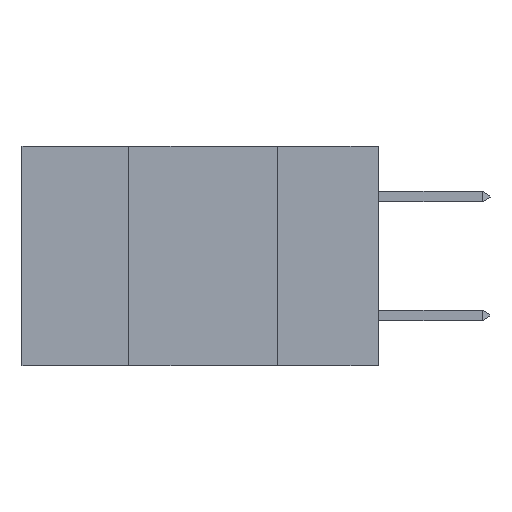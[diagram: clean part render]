
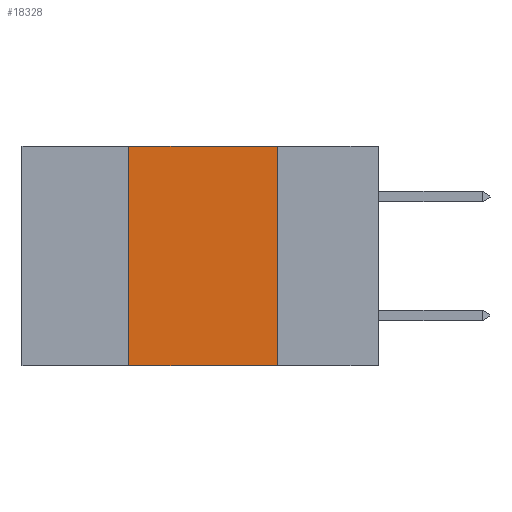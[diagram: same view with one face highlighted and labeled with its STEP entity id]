
A CAD part, left-side view. The second image highlights one B-rep face of the part: STEP entity #18328.
In plain terms, the highlighted planar face has unit normal (-1, 0, 0).
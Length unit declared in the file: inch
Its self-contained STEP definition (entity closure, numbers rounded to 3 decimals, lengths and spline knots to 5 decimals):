
#349 = LINE ( 'NONE', #16139, #8867 ) ;
#1029 = CARTESIAN_POINT ( 'NONE',  ( 0., 0.42, 0. ) ) ;
#1125 = AXIS2_PLACEMENT_3D ( 'NONE', #12153, #16724, #7629 ) ;
#2947 = EDGE_CURVE ( 'NONE', #4240, #19708, #18165, .T. ) ;
#3230 = VERTEX_POINT ( 'NONE', #1029 ) ;
#3625 = CARTESIAN_POINT ( 'NONE',  ( 0., 0.17, -0.37 ) ) ;
#4240 = VERTEX_POINT ( 'NONE', #11007 ) ;
#5170 = EDGE_CURVE ( 'NONE', #18946, #3230, #349, .T. ) ;
#7629 = DIRECTION ( 'NONE',  ( 0., 0., -1. ) ) ;
#8013 = VECTOR ( 'NONE', #11892, 39.37008 ) ;
#8538 = EDGE_CURVE ( 'NONE', #18946, #19708, #20513, .T. ) ;
#8867 = VECTOR ( 'NONE', #19160, 39.37008 ) ;
#9620 = VECTOR ( 'NONE', #17182, 39.37008 ) ;
#11007 = CARTESIAN_POINT ( 'NONE',  ( 0., 0.17, 0. ) ) ;
#11129 = ORIENTED_EDGE ( 'NONE', *, *, #8538, .T. ) ;
#11775 = EDGE_CURVE ( 'NONE', #3230, #4240, #16071, .T. ) ;
#11892 = DIRECTION ( 'NONE',  ( 0., -1., 0. ) ) ;
#12153 = CARTESIAN_POINT ( 'NONE',  ( 0., 0.6, 0. ) ) ;
#12509 = VECTOR ( 'NONE', #17464, 39.37008 ) ;
#13045 = ORIENTED_EDGE ( 'NONE', *, *, #2947, .F. ) ;
#13361 = CARTESIAN_POINT ( 'NONE',  ( 0., 0.6, 0. ) ) ;
#14089 = EDGE_LOOP ( 'NONE', ( #13045, #15999, #15626, #11129 ) ) ;
#15161 = PLANE ( 'NONE',  #1125 ) ;
#15262 = CARTESIAN_POINT ( 'NONE',  ( 0., 0.17, 0. ) ) ;
#15626 = ORIENTED_EDGE ( 'NONE', *, *, #5170, .F. ) ;
#15909 = CARTESIAN_POINT ( 'NONE',  ( 0., 0.6, -0.37 ) ) ;
#15999 = ORIENTED_EDGE ( 'NONE', *, *, #11775, .F. ) ;
#16071 = LINE ( 'NONE', #13361, #8013 ) ;
#16139 = CARTESIAN_POINT ( 'NONE',  ( 0., 0.42, 0. ) ) ;
#16198 = CARTESIAN_POINT ( 'NONE',  ( 0., 0.42, -0.37 ) ) ;
#16724 = DIRECTION ( 'NONE',  ( 1., 0., 0. ) ) ;
#17182 = DIRECTION ( 'NONE',  ( 0., 0., -1. ) ) ;
#17464 = DIRECTION ( 'NONE',  ( 0., -1., 0. ) ) ;
#18165 = LINE ( 'NONE', #15262, #9620 ) ;
#18328 = ADVANCED_FACE ( 'NONE', ( #19063 ), #15161, .F. ) ;
#18946 = VERTEX_POINT ( 'NONE', #16198 ) ;
#19063 = FACE_OUTER_BOUND ( 'NONE', #14089, .T. ) ;
#19160 = DIRECTION ( 'NONE',  ( 0., 0., 1. ) ) ;
#19708 = VERTEX_POINT ( 'NONE', #3625 ) ;
#20513 = LINE ( 'NONE', #15909, #12509 ) ;
